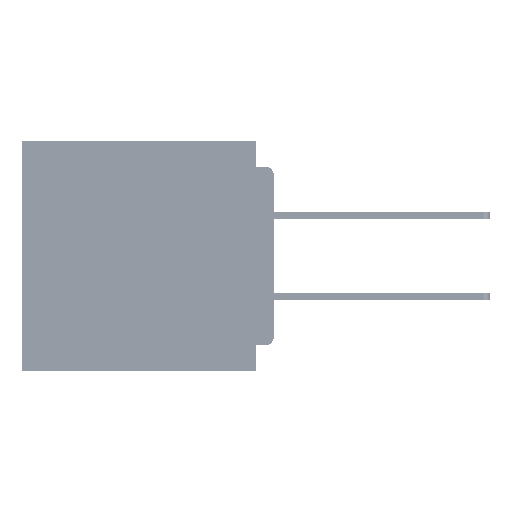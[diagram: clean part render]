
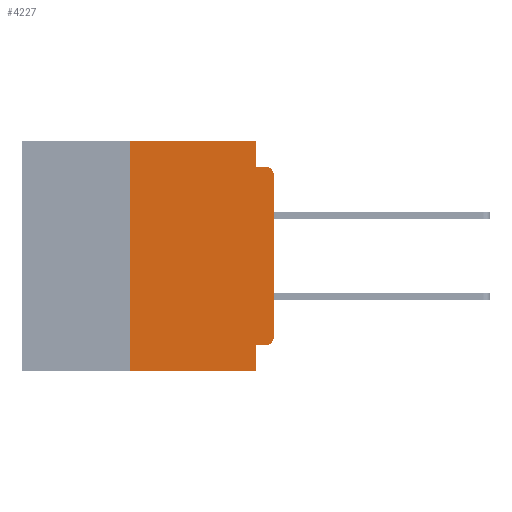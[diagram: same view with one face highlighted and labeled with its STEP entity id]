
A CAD part, left-side view. The second image highlights one B-rep face of the part: STEP entity #4227.
In plain terms, the highlighted planar face has unit normal (-1, 0, 0).
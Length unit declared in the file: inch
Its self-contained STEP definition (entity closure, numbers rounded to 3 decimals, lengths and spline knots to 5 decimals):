
#222 = DIRECTION ( 'NONE',  ( 1., 0., 0. ) ) ;
#743 = EDGE_CURVE ( 'NONE', #45928, #29902, #62453, .T. ) ;
#1632 = VECTOR ( 'NONE', #55957, 39.37008 ) ;
#1694 = LINE ( 'NONE', #34120, #25516 ) ;
#1842 = CARTESIAN_POINT ( 'NONE',  ( 0., 0., -0.355 ) ) ;
#2482 = VECTOR ( 'NONE', #20845, 39.37008 ) ;
#3375 = VERTEX_POINT ( 'NONE', #19875 ) ;
#3754 = CARTESIAN_POINT ( 'NONE',  ( 0., 0.437, 0. ) ) ;
#4078 = ORIENTED_EDGE ( 'NONE', *, *, #54812, .F. ) ;
#4179 = LINE ( 'NONE', #31720, #2482 ) ;
#4227 = ADVANCED_FACE ( 'NONE', ( #50102 ), #65247, .F. ) ;
#4443 = VERTEX_POINT ( 'NONE', #34174 ) ;
#8125 = CARTESIAN_POINT ( 'NONE',  ( 0., 0., -0.34 ) ) ;
#8626 = CARTESIAN_POINT ( 'NONE',  ( 0., 0.437, -0.4 ) ) ;
#9003 = DIRECTION ( 'NONE',  ( -1., 0., 0. ) ) ;
#9512 = VECTOR ( 'NONE', #61525, 39.37008 ) ;
#9931 = VERTEX_POINT ( 'NONE', #57788 ) ;
#10033 = CARTESIAN_POINT ( 'NONE',  ( 0., 0.25, -0.4 ) ) ;
#11230 = LINE ( 'NONE', #18164, #9512 ) ;
#11881 = EDGE_CURVE ( 'NONE', #65903, #48808, #58875, .T. ) ;
#11994 = EDGE_CURVE ( 'NONE', #29902, #3375, #53739, .T. ) ;
#15108 = VECTOR ( 'NONE', #65069, 39.37008 ) ;
#15949 = VERTEX_POINT ( 'NONE', #56216 ) ;
#16107 = EDGE_CURVE ( 'NONE', #4443, #39596, #21197, .T. ) ;
#16811 = LINE ( 'NONE', #8626, #29492 ) ;
#18164 = CARTESIAN_POINT ( 'NONE',  ( 0., 0.031, -0.4 ) ) ;
#19875 = CARTESIAN_POINT ( 'NONE',  ( 0., 0.031, 0. ) ) ;
#20845 = DIRECTION ( 'NONE',  ( 0., 0., 1. ) ) ;
#21197 = CIRCLE ( 'NONE', #50348, 0.015 ) ;
#21904 = CARTESIAN_POINT ( 'NONE',  ( 0., 0.437, 0. ) ) ;
#24204 = EDGE_CURVE ( 'NONE', #45928, #9931, #16811, .T. ) ;
#24691 = CARTESIAN_POINT ( 'NONE',  ( 0., 0.015, -0.06 ) ) ;
#25278 = ORIENTED_EDGE ( 'NONE', *, *, #16107, .T. ) ;
#25516 = VECTOR ( 'NONE', #28925, 39.37008 ) ;
#25723 = AXIS2_PLACEMENT_3D ( 'NONE', #24691, #62603, #30128 ) ;
#27137 = CARTESIAN_POINT ( 'NONE',  ( 0., 0., -0.045 ) ) ;
#28925 = DIRECTION ( 'NONE',  ( 0., 0., -1. ) ) ;
#29162 = EDGE_CURVE ( 'NONE', #39596, #65903, #4179, .T. ) ;
#29492 = VECTOR ( 'NONE', #68103, 39.37008 ) ;
#29902 = VERTEX_POINT ( 'NONE', #37985 ) ;
#30128 = DIRECTION ( 'NONE',  ( 0., 0., -1. ) ) ;
#30805 = DIRECTION ( 'NONE',  ( 0., -1., 0. ) ) ;
#31720 = CARTESIAN_POINT ( 'NONE',  ( 0., 0., 0. ) ) ;
#33033 = AXIS2_PLACEMENT_3D ( 'NONE', #21904, #222, #38193 ) ;
#33598 = VECTOR ( 'NONE', #43103, 39.37008 ) ;
#34120 = CARTESIAN_POINT ( 'NONE',  ( 0., 0.031, 0. ) ) ;
#34174 = CARTESIAN_POINT ( 'NONE',  ( 0., 0.015, -0.355 ) ) ;
#34936 = ORIENTED_EDGE ( 'NONE', *, *, #11881, .T. ) ;
#35118 = CARTESIAN_POINT ( 'NONE',  ( 0., 0., -0.06 ) ) ;
#37681 = CARTESIAN_POINT ( 'NONE',  ( 0., 0.25, -0.4 ) ) ;
#37985 = CARTESIAN_POINT ( 'NONE',  ( 0., 0.25, 0. ) ) ;
#38193 = DIRECTION ( 'NONE',  ( 0., 0., -1. ) ) ;
#39596 = VERTEX_POINT ( 'NONE', #8125 ) ;
#41393 = CARTESIAN_POINT ( 'NONE',  ( 0., 0.015, -0.34 ) ) ;
#42250 = EDGE_CURVE ( 'NONE', #4443, #15949, #50014, .T. ) ;
#43103 = DIRECTION ( 'NONE',  ( 0., 0., 1. ) ) ;
#44973 = CARTESIAN_POINT ( 'NONE',  ( 0., 0.015, -0.045 ) ) ;
#45928 = VERTEX_POINT ( 'NONE', #10033 ) ;
#46842 = EDGE_CURVE ( 'NONE', #3375, #54208, #1694, .T. ) ;
#46870 = DIRECTION ( 'NONE',  ( 0., 0., -1. ) ) ;
#48433 = ORIENTED_EDGE ( 'NONE', *, *, #29162, .T. ) ;
#48808 = VERTEX_POINT ( 'NONE', #44973 ) ;
#50014 = LINE ( 'NONE', #1842, #1632 ) ;
#50102 = FACE_OUTER_BOUND ( 'NONE', #69611, .T. ) ;
#50348 = AXIS2_PLACEMENT_3D ( 'NONE', #41393, #9003, #46870 ) ;
#53304 = ORIENTED_EDGE ( 'NONE', *, *, #743, .F. ) ;
#53739 = LINE ( 'NONE', #3754, #64772 ) ;
#54066 = ORIENTED_EDGE ( 'NONE', *, *, #42250, .F. ) ;
#54208 = VERTEX_POINT ( 'NONE', #66825 ) ;
#54812 = EDGE_CURVE ( 'NONE', #15949, #9931, #11230, .T. ) ;
#55370 = ORIENTED_EDGE ( 'NONE', *, *, #46842, .F. ) ;
#55957 = DIRECTION ( 'NONE',  ( 0., 1., 0. ) ) ;
#56216 = CARTESIAN_POINT ( 'NONE',  ( 0., 0.031, -0.355 ) ) ;
#57780 = ORIENTED_EDGE ( 'NONE', *, *, #69888, .F. ) ;
#57788 = CARTESIAN_POINT ( 'NONE',  ( 0., 0.031, -0.4 ) ) ;
#58328 = LINE ( 'NONE', #27137, #15108 ) ;
#58875 = CIRCLE ( 'NONE', #25723, 0.015 ) ;
#61525 = DIRECTION ( 'NONE',  ( 0., 0., -1. ) ) ;
#62453 = LINE ( 'NONE', #37681, #33598 ) ;
#62603 = DIRECTION ( 'NONE',  ( -1., 0., 0. ) ) ;
#64587 = ORIENTED_EDGE ( 'NONE', *, *, #11994, .F. ) ;
#64772 = VECTOR ( 'NONE', #30805, 39.37008 ) ;
#65069 = DIRECTION ( 'NONE',  ( 0., -1., 0. ) ) ;
#65247 = PLANE ( 'NONE',  #33033 ) ;
#65903 = VERTEX_POINT ( 'NONE', #35118 ) ;
#66444 = ORIENTED_EDGE ( 'NONE', *, *, #24204, .T. ) ;
#66825 = CARTESIAN_POINT ( 'NONE',  ( 0., 0.031, -0.045 ) ) ;
#68103 = DIRECTION ( 'NONE',  ( 0., -1., 0. ) ) ;
#69611 = EDGE_LOOP ( 'NONE', ( #48433, #34936, #57780, #55370, #64587, #53304, #66444, #4078, #54066, #25278 ) ) ;
#69888 = EDGE_CURVE ( 'NONE', #54208, #48808, #58328, .T. ) ;
